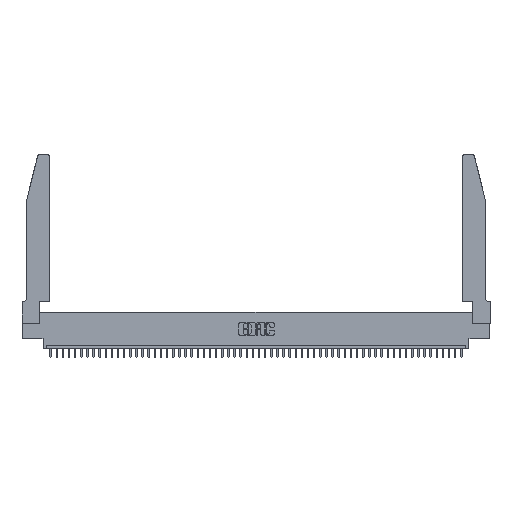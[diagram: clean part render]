
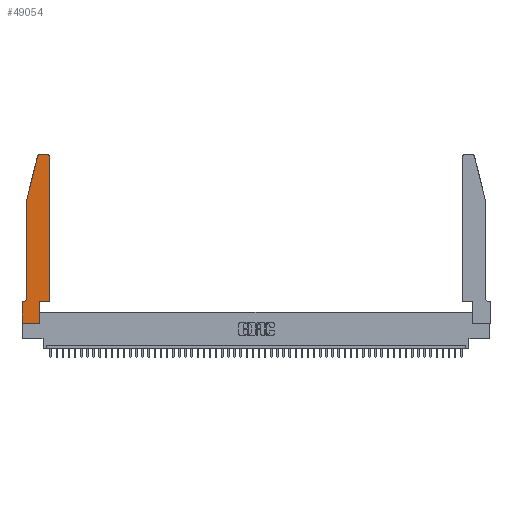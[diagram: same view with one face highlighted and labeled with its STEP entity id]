
A CAD part, top view. The second image highlights one B-rep face of the part: STEP entity #49054.
In plain terms, the highlighted planar face has unit normal (0, 0, 1).
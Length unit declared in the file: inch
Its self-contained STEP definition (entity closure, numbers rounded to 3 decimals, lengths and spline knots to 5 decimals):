
#90 = EDGE_CURVE ( 'NONE', #29832, #12241, #43046, .T. ) ;
#1053 = CARTESIAN_POINT ( 'NONE',  ( 0., 0., 0.37 ) ) ;
#1380 = CARTESIAN_POINT ( 'NONE',  ( 0.25487, 2.72718, 0.37 ) ) ;
#1940 = DIRECTION ( 'NONE',  ( -0.239, -0.971, 0. ) ) ;
#2113 = VERTEX_POINT ( 'NONE', #14644 ) ;
#2177 = EDGE_CURVE ( 'NONE', #39444, #14777, #45371, .T. ) ;
#3792 = VECTOR ( 'NONE', #10434, 39.37008 ) ;
#3948 = DIRECTION ( 'NONE',  ( -1., 0., 0. ) ) ;
#4508 = EDGE_CURVE ( 'NONE', #28761, #19443, #20934, .T. ) ;
#5447 = CIRCLE ( 'NONE', #18486, 0.03 ) ;
#6554 = LINE ( 'NONE', #46697, #40902 ) ;
#7051 = AXIS2_PLACEMENT_3D ( 'NONE', #11878, #15623, #24279 ) ;
#8993 = CARTESIAN_POINT ( 'NONE',  ( 0., 0., 0.37 ) ) ;
#9240 = LINE ( 'NONE', #38956, #41083 ) ;
#10054 = VERTEX_POINT ( 'NONE', #1380 ) ;
#10393 = CARTESIAN_POINT ( 'NONE',  ( 0.2605, 2.75, 0.37 ) ) ;
#10434 = DIRECTION ( 'NONE',  ( 0., -1., 0. ) ) ;
#10736 = CARTESIAN_POINT ( 'NONE',  ( 0., 0.35, 0.37 ) ) ;
#11878 = CARTESIAN_POINT ( 'NONE',  ( 0., 0.35, 0.37 ) ) ;
#12163 = EDGE_LOOP ( 'NONE', ( #33105, #15534, #14590, #32083, #46769, #13792, #13510, #25507, #49502, #34567, #43477, #26218 ) ) ;
#12241 = VERTEX_POINT ( 'NONE', #22141 ) ;
#13510 = ORIENTED_EDGE ( 'NONE', *, *, #4508, .T. ) ;
#13628 = CARTESIAN_POINT ( 'NONE',  ( 0.4205, 2.72, 0.37 ) ) ;
#13667 = CARTESIAN_POINT ( 'NONE',  ( 0.2865, 0., 0.37 ) ) ;
#13792 = ORIENTED_EDGE ( 'NONE', *, *, #39214, .T. ) ;
#13819 = DIRECTION ( 'NONE',  ( 1., 0., 0. ) ) ;
#13963 = DIRECTION ( 'NONE',  ( 0., 1., 0. ) ) ;
#14301 = DIRECTION ( 'NONE',  ( -1., 0., 0. ) ) ;
#14590 = ORIENTED_EDGE ( 'NONE', *, *, #15364, .T. ) ;
#14644 = CARTESIAN_POINT ( 'NONE',  ( 0.0755, 0.42, 0.37 ) ) ;
#14696 = DIRECTION ( 'NONE',  ( 0., 0., 1. ) ) ;
#14777 = VERTEX_POINT ( 'NONE', #15755 ) ;
#15111 = EDGE_CURVE ( 'NONE', #15711, #10054, #5447, .T. ) ;
#15132 = CARTESIAN_POINT ( 'NONE',  ( 0.284, 2.75, 0.37 ) ) ;
#15364 = EDGE_CURVE ( 'NONE', #10054, #20508, #9240, .T. ) ;
#15522 = CARTESIAN_POINT ( 'NONE',  ( 0.0055, 0.42, 0.37 ) ) ;
#15534 = ORIENTED_EDGE ( 'NONE', *, *, #15111, .T. ) ;
#15623 = DIRECTION ( 'NONE',  ( 0., 0., 1. ) ) ;
#15711 = VERTEX_POINT ( 'NONE', #15132 ) ;
#15755 = CARTESIAN_POINT ( 'NONE',  ( 0.4505, 0.35, 0.37 ) ) ;
#16109 = FACE_OUTER_BOUND ( 'NONE', #12163, .T. ) ;
#16156 = EDGE_CURVE ( 'NONE', #12241, #15711, #47414, .T. ) ;
#16952 = CIRCLE ( 'NONE', #34439, 0.07 ) ;
#17467 = VECTOR ( 'NONE', #14301, 39.37008 ) ;
#17502 = LINE ( 'NONE', #43418, #28358 ) ;
#18005 = CARTESIAN_POINT ( 'NONE',  ( 0.0055, 0.35, 0.37 ) ) ;
#18486 = AXIS2_PLACEMENT_3D ( 'NONE', #42960, #14696, #30513 ) ;
#19109 = DIRECTION ( 'NONE',  ( 0., -1., 0. ) ) ;
#19443 = VERTEX_POINT ( 'NONE', #1053 ) ;
#20508 = VERTEX_POINT ( 'NONE', #42655 ) ;
#20934 = LINE ( 'NONE', #8993, #3792 ) ;
#22141 = CARTESIAN_POINT ( 'NONE',  ( 0.4205, 2.75, 0.37 ) ) ;
#24279 = DIRECTION ( 'NONE',  ( 1., 0., 0. ) ) ;
#24766 = LINE ( 'NONE', #40412, #47744 ) ;
#25169 = EDGE_CURVE ( 'NONE', #2113, #30994, #16952, .T. ) ;
#25507 = ORIENTED_EDGE ( 'NONE', *, *, #41610, .T. ) ;
#26218 = ORIENTED_EDGE ( 'NONE', *, *, #90, .T. ) ;
#27602 = CARTESIAN_POINT ( 'NONE',  ( 0.2865, 0.35, 0.37 ) ) ;
#28358 = VECTOR ( 'NONE', #48004, 39.37008 ) ;
#28761 = VERTEX_POINT ( 'NONE', #10736 ) ;
#29832 = VERTEX_POINT ( 'NONE', #48584 ) ;
#30513 = DIRECTION ( 'NONE',  ( 1., 0., 0. ) ) ;
#30994 = VERTEX_POINT ( 'NONE', #18005 ) ;
#32083 = ORIENTED_EDGE ( 'NONE', *, *, #33518, .T. ) ;
#32660 = AXIS2_PLACEMENT_3D ( 'NONE', #13628, #45187, #50818 ) ;
#32696 = VECTOR ( 'NONE', #13819, 39.37008 ) ;
#33105 = ORIENTED_EDGE ( 'NONE', *, *, #16156, .T. ) ;
#33518 = EDGE_CURVE ( 'NONE', #20508, #2113, #35907, .T. ) ;
#33641 = LINE ( 'NONE', #50544, #49513 ) ;
#34439 = AXIS2_PLACEMENT_3D ( 'NONE', #15522, #52247, #3948 ) ;
#34567 = ORIENTED_EDGE ( 'NONE', *, *, #2177, .T. ) ;
#35907 = LINE ( 'NONE', #39213, #51142 ) ;
#38956 = CARTESIAN_POINT ( 'NONE',  ( 0.0755, 2., 0.37 ) ) ;
#39213 = CARTESIAN_POINT ( 'NONE',  ( 0.0755, 2., 0.37 ) ) ;
#39214 = EDGE_CURVE ( 'NONE', #30994, #28761, #24766, .T. ) ;
#39444 = VERTEX_POINT ( 'NONE', #27602 ) ;
#40412 = CARTESIAN_POINT ( 'NONE',  ( 0.0755, 0.35, 0.37 ) ) ;
#40902 = VECTOR ( 'NONE', #13963, 39.37008 ) ;
#41083 = VECTOR ( 'NONE', #1940, 39.37008 ) ;
#41610 = EDGE_CURVE ( 'NONE', #19443, #45417, #17502, .T. ) ;
#42413 = DIRECTION ( 'NONE',  ( 0., 1., 0. ) ) ;
#42655 = CARTESIAN_POINT ( 'NONE',  ( 0.0755, 2., 0.37 ) ) ;
#42960 = CARTESIAN_POINT ( 'NONE',  ( 0.284, 2.72, 0.37 ) ) ;
#43046 = CIRCLE ( 'NONE', #32660, 0.03 ) ;
#43418 = CARTESIAN_POINT ( 'NONE',  ( 0., 0., 0.37 ) ) ;
#43477 = ORIENTED_EDGE ( 'NONE', *, *, #52499, .T. ) ;
#43989 = DIRECTION ( 'NONE',  ( -1., 0., 0. ) ) ;
#44407 = PLANE ( 'NONE',  #7051 ) ;
#44970 = CARTESIAN_POINT ( 'NONE',  ( 0.4505, 0.35, 0.37 ) ) ;
#45187 = DIRECTION ( 'NONE',  ( 0., 0., 1. ) ) ;
#45371 = LINE ( 'NONE', #44970, #32696 ) ;
#45417 = VERTEX_POINT ( 'NONE', #13667 ) ;
#46697 = CARTESIAN_POINT ( 'NONE',  ( 0.2865, 0.35, 0.37 ) ) ;
#46769 = ORIENTED_EDGE ( 'NONE', *, *, #25169, .T. ) ;
#47414 = LINE ( 'NONE', #10393, #17467 ) ;
#47744 = VECTOR ( 'NONE', #43989, 39.37008 ) ;
#48004 = DIRECTION ( 'NONE',  ( 1., 0., 0. ) ) ;
#48584 = CARTESIAN_POINT ( 'NONE',  ( 0.4505, 2.72, 0.37 ) ) ;
#49054 = ADVANCED_FACE ( 'NONE', ( #16109 ), #44407, .T. ) ;
#49502 = ORIENTED_EDGE ( 'NONE', *, *, #50633, .T. ) ;
#49513 = VECTOR ( 'NONE', #42413, 39.37008 ) ;
#50544 = CARTESIAN_POINT ( 'NONE',  ( 0.4505, 0.35, 0.37 ) ) ;
#50633 = EDGE_CURVE ( 'NONE', #45417, #39444, #6554, .T. ) ;
#50818 = DIRECTION ( 'NONE',  ( 1., 0., 0. ) ) ;
#51142 = VECTOR ( 'NONE', #19109, 39.37008 ) ;
#52247 = DIRECTION ( 'NONE',  ( 0., 0., -1. ) ) ;
#52499 = EDGE_CURVE ( 'NONE', #14777, #29832, #33641, .T. ) ;
